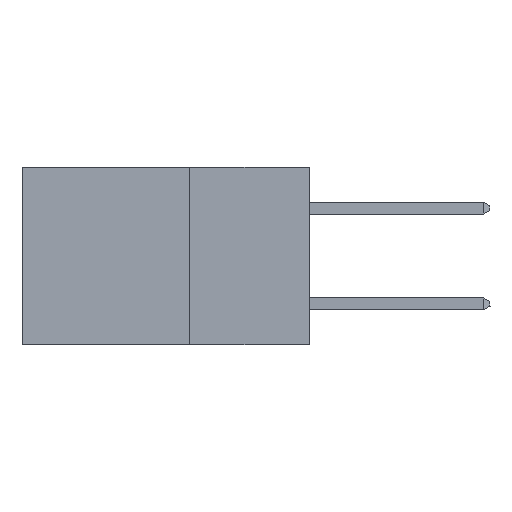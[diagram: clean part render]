
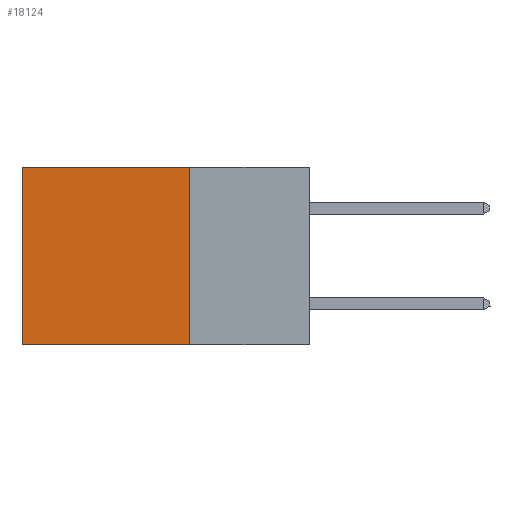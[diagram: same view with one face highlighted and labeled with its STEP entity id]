
A CAD part, left-side view. The second image highlights one B-rep face of the part: STEP entity #18124.
In plain terms, the highlighted planar face has unit normal (-1, 0, 0).
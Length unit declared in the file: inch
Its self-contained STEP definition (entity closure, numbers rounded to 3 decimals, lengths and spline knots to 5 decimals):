
#883 = CARTESIAN_POINT ( 'NONE',  ( 0.2875, 0.25, 0. ) ) ;
#1568 = VECTOR ( 'NONE', #6875, 39.37008 ) ;
#3579 = CARTESIAN_POINT ( 'NONE',  ( 0.2875, 0.6, -0.37 ) ) ;
#4195 = VERTEX_POINT ( 'NONE', #3579 ) ;
#4900 = LINE ( 'NONE', #21422, #6921 ) ;
#5061 = EDGE_CURVE ( 'NONE', #9785, #4195, #27661, .T. ) ;
#5420 = VERTEX_POINT ( 'NONE', #883 ) ;
#5963 = DIRECTION ( 'NONE',  ( 0., 1., 0. ) ) ;
#6196 = EDGE_CURVE ( 'NONE', #5420, #20139, #6228, .T. ) ;
#6228 = LINE ( 'NONE', #19863, #1568 ) ;
#6875 = DIRECTION ( 'NONE',  ( 0., 0., -1. ) ) ;
#6921 = VECTOR ( 'NONE', #15038, 39.37008 ) ;
#7515 = EDGE_LOOP ( 'NONE', ( #22385, #15052, #16554, #26559 ) ) ;
#8454 = AXIS2_PLACEMENT_3D ( 'NONE', #25304, #25399, #12262 ) ;
#9785 = VERTEX_POINT ( 'NONE', #15439 ) ;
#10094 = VECTOR ( 'NONE', #5963, 39.37008 ) ;
#12018 = EDGE_CURVE ( 'NONE', #5420, #9785, #4900, .T. ) ;
#12262 = DIRECTION ( 'NONE',  ( 0., 0., -1. ) ) ;
#12289 = CARTESIAN_POINT ( 'NONE',  ( 0.2875, 0.25, -0.37 ) ) ;
#12865 = VECTOR ( 'NONE', #27068, 39.37008 ) ;
#15038 = DIRECTION ( 'NONE',  ( 0., 1., 0. ) ) ;
#15052 = ORIENTED_EDGE ( 'NONE', *, *, #23767, .F. ) ;
#15439 = CARTESIAN_POINT ( 'NONE',  ( 0.2875, 0.6, 0. ) ) ;
#16554 = ORIENTED_EDGE ( 'NONE', *, *, #6196, .F. ) ;
#18124 = ADVANCED_FACE ( 'NONE', ( #22424 ), #18646, .F. ) ;
#18442 = CARTESIAN_POINT ( 'NONE',  ( 0.2875, 0.25, -0.37 ) ) ;
#18646 = PLANE ( 'NONE',  #8454 ) ;
#19863 = CARTESIAN_POINT ( 'NONE',  ( 0.2875, 0.25, 0. ) ) ;
#20139 = VERTEX_POINT ( 'NONE', #18442 ) ;
#21422 = CARTESIAN_POINT ( 'NONE',  ( 0.2875, 0.25, 0. ) ) ;
#22385 = ORIENTED_EDGE ( 'NONE', *, *, #5061, .T. ) ;
#22424 = FACE_OUTER_BOUND ( 'NONE', #7515, .T. ) ;
#23767 = EDGE_CURVE ( 'NONE', #20139, #4195, #26822, .T. ) ;
#24546 = CARTESIAN_POINT ( 'NONE',  ( 0.2875, 0.6, 0. ) ) ;
#25304 = CARTESIAN_POINT ( 'NONE',  ( 0.2875, 0.25, 0. ) ) ;
#25399 = DIRECTION ( 'NONE',  ( 1., 0., 0. ) ) ;
#26559 = ORIENTED_EDGE ( 'NONE', *, *, #12018, .T. ) ;
#26822 = LINE ( 'NONE', #12289, #10094 ) ;
#27068 = DIRECTION ( 'NONE',  ( 0., 0., -1. ) ) ;
#27661 = LINE ( 'NONE', #24546, #12865 ) ;
